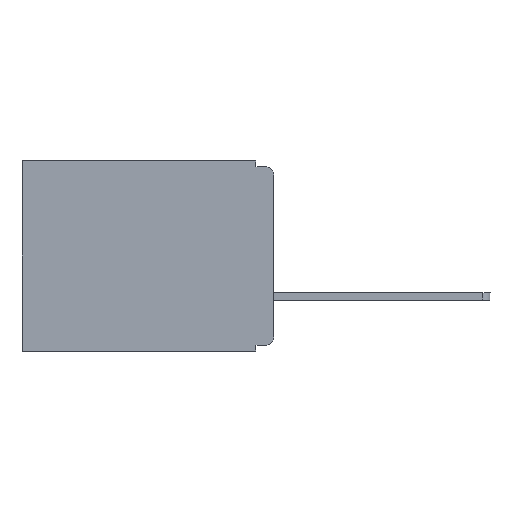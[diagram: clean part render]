
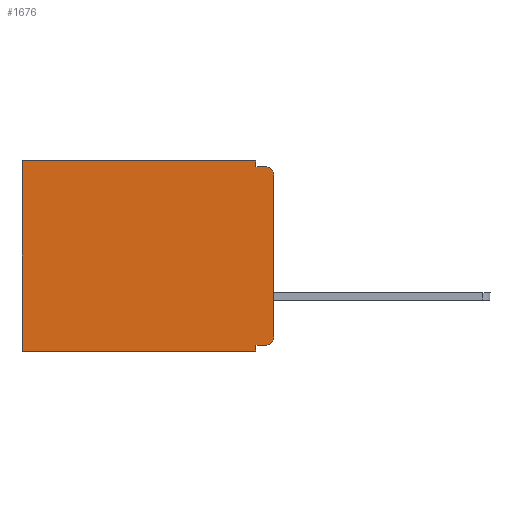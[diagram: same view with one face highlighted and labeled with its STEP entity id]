
A CAD part, left-side view. The second image highlights one B-rep face of the part: STEP entity #1676.
In plain terms, the highlighted planar face has unit normal (-1, 0, 0).
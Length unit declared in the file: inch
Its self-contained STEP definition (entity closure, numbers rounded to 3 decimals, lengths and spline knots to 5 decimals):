
#54 = CARTESIAN_POINT ( 'NONE',  ( 0.3, 0., -0.33 ) ) ;
#167 = VERTEX_POINT ( 'NONE', #6748 ) ;
#333 = VECTOR ( 'NONE', #10837, 39.37008 ) ;
#341 = PLANE ( 'NONE',  #2718 ) ;
#878 = DIRECTION ( 'NONE',  ( 0., 1., 0. ) ) ;
#884 = VECTOR ( 'NONE', #2899, 39.37008 ) ;
#930 = EDGE_CURVE ( 'NONE', #6573, #12989, #11190, .T. ) ;
#1018 = ORIENTED_EDGE ( 'NONE', *, *, #9528, .T. ) ;
#1331 = VERTEX_POINT ( 'NONE', #4767 ) ;
#1585 = EDGE_CURVE ( 'NONE', #167, #3086, #12884, .T. ) ;
#1676 = ADVANCED_FACE ( 'NONE', ( #2302 ), #341, .F. ) ;
#2039 = ORIENTED_EDGE ( 'NONE', *, *, #930, .T. ) ;
#2302 = FACE_OUTER_BOUND ( 'NONE', #2448, .T. ) ;
#2439 = CIRCLE ( 'NONE', #5686, 0.015 ) ;
#2448 = EDGE_LOOP ( 'NONE', ( #11182, #5757, #12698, #13178, #2039, #1018, #11456, #3758, #7376, #3087 ) ) ;
#2454 = LINE ( 'NONE', #13565, #10683 ) ;
#2503 = EDGE_CURVE ( 'NONE', #13521, #1331, #2439, .T. ) ;
#2718 = AXIS2_PLACEMENT_3D ( 'NONE', #3379, #8680, #5554 ) ;
#2777 = DIRECTION ( 'NONE',  ( 0., 1., 0. ) ) ;
#2899 = DIRECTION ( 'NONE',  ( 0., -1., 0. ) ) ;
#3066 = AXIS2_PLACEMENT_3D ( 'NONE', #4634, #8863, #5655 ) ;
#3086 = VERTEX_POINT ( 'NONE', #11547 ) ;
#3087 = ORIENTED_EDGE ( 'NONE', *, *, #10716, .T. ) ;
#3252 = VERTEX_POINT ( 'NONE', #3298 ) ;
#3274 = CARTESIAN_POINT ( 'NONE',  ( 0.3, 0., -0.32 ) ) ;
#3298 = CARTESIAN_POINT ( 'NONE',  ( 0.3, 0., -0.305 ) ) ;
#3379 = CARTESIAN_POINT ( 'NONE',  ( 0.3, 0., -0.33 ) ) ;
#3758 = ORIENTED_EDGE ( 'NONE', *, *, #9225, .F. ) ;
#3961 = DIRECTION ( 'NONE',  ( 0., 0., -1. ) ) ;
#4039 = VECTOR ( 'NONE', #7581, 39.37008 ) ;
#4058 = EDGE_CURVE ( 'NONE', #9631, #13279, #10484, .T. ) ;
#4242 = CARTESIAN_POINT ( 'NONE',  ( 0.3, 0.015, -0.32 ) ) ;
#4634 = CARTESIAN_POINT ( 'NONE',  ( 0.3, 0.015, -0.305 ) ) ;
#4767 = CARTESIAN_POINT ( 'NONE',  ( 0.3, 0.015, -0.01 ) ) ;
#5142 = DIRECTION ( 'NONE',  ( 0., 0., -1. ) ) ;
#5554 = DIRECTION ( 'NONE',  ( 0., 0., -1. ) ) ;
#5655 = DIRECTION ( 'NONE',  ( 0., 0., -1. ) ) ;
#5686 = AXIS2_PLACEMENT_3D ( 'NONE', #9345, #12616, #5142 ) ;
#5718 = LINE ( 'NONE', #9751, #333 ) ;
#5719 = EDGE_CURVE ( 'NONE', #13521, #3252, #5801, .T. ) ;
#5757 = ORIENTED_EDGE ( 'NONE', *, *, #2503, .T. ) ;
#5801 = LINE ( 'NONE', #12309, #12481 ) ;
#6573 = VERTEX_POINT ( 'NONE', #9474 ) ;
#6748 = CARTESIAN_POINT ( 'NONE',  ( 0.3, 0.031, -0.33 ) ) ;
#7028 = CARTESIAN_POINT ( 'NONE',  ( 0.3, 0., 0. ) ) ;
#7119 = CARTESIAN_POINT ( 'NONE',  ( 0.3, 0.031, -0.33 ) ) ;
#7376 = ORIENTED_EDGE ( 'NONE', *, *, #4058, .F. ) ;
#7581 = DIRECTION ( 'NONE',  ( 0., 1., 0. ) ) ;
#7694 = VECTOR ( 'NONE', #10403, 39.37008 ) ;
#8056 = EDGE_CURVE ( 'NONE', #11805, #1331, #10870, .T. ) ;
#8240 = VECTOR ( 'NONE', #2777, 39.37008 ) ;
#8373 = CIRCLE ( 'NONE', #3066, 0.015 ) ;
#8680 = DIRECTION ( 'NONE',  ( 1., 0., 0. ) ) ;
#8752 = CARTESIAN_POINT ( 'NONE',  ( 0.3, 0.437, 0. ) ) ;
#8863 = DIRECTION ( 'NONE',  ( -1., 0., 0. ) ) ;
#9077 = DIRECTION ( 'NONE',  ( 0., 0., -1. ) ) ;
#9225 = EDGE_CURVE ( 'NONE', #13279, #167, #12386, .T. ) ;
#9345 = CARTESIAN_POINT ( 'NONE',  ( 0.3, 0.015, -0.025 ) ) ;
#9474 = CARTESIAN_POINT ( 'NONE',  ( 0.3, 0.031, 0. ) ) ;
#9528 = EDGE_CURVE ( 'NONE', #12989, #3086, #2454, .T. ) ;
#9631 = VERTEX_POINT ( 'NONE', #4242 ) ;
#9751 = CARTESIAN_POINT ( 'NONE',  ( 0.3, 0.031, 0. ) ) ;
#10403 = DIRECTION ( 'NONE',  ( 0., 0., -1. ) ) ;
#10484 = LINE ( 'NONE', #3274, #4039 ) ;
#10683 = VECTOR ( 'NONE', #3961, 39.37008 ) ;
#10691 = EDGE_CURVE ( 'NONE', #6573, #11805, #5718, .T. ) ;
#10716 = EDGE_CURVE ( 'NONE', #9631, #3252, #8373, .T. ) ;
#10837 = DIRECTION ( 'NONE',  ( 0., 0., -1. ) ) ;
#10870 = LINE ( 'NONE', #13680, #884 ) ;
#11182 = ORIENTED_EDGE ( 'NONE', *, *, #5719, .F. ) ;
#11190 = LINE ( 'NONE', #7028, #8240 ) ;
#11456 = ORIENTED_EDGE ( 'NONE', *, *, #1585, .F. ) ;
#11547 = CARTESIAN_POINT ( 'NONE',  ( 0.3, 0.437, -0.33 ) ) ;
#11805 = VERTEX_POINT ( 'NONE', #13422 ) ;
#12309 = CARTESIAN_POINT ( 'NONE',  ( 0.3, 0., -0.33 ) ) ;
#12386 = LINE ( 'NONE', #7119, #7694 ) ;
#12481 = VECTOR ( 'NONE', #9077, 39.37008 ) ;
#12554 = VECTOR ( 'NONE', #878, 39.37008 ) ;
#12616 = DIRECTION ( 'NONE',  ( -1., 0., 0. ) ) ;
#12698 = ORIENTED_EDGE ( 'NONE', *, *, #8056, .F. ) ;
#12729 = CARTESIAN_POINT ( 'NONE',  ( 0.3, 0., -0.025 ) ) ;
#12742 = CARTESIAN_POINT ( 'NONE',  ( 0.3, 0.031, -0.32 ) ) ;
#12884 = LINE ( 'NONE', #54, #12554 ) ;
#12989 = VERTEX_POINT ( 'NONE', #8752 ) ;
#13178 = ORIENTED_EDGE ( 'NONE', *, *, #10691, .F. ) ;
#13279 = VERTEX_POINT ( 'NONE', #12742 ) ;
#13422 = CARTESIAN_POINT ( 'NONE',  ( 0.3, 0.031, -0.01 ) ) ;
#13521 = VERTEX_POINT ( 'NONE', #12729 ) ;
#13565 = CARTESIAN_POINT ( 'NONE',  ( 0.3, 0.437, -0.33 ) ) ;
#13680 = CARTESIAN_POINT ( 'NONE',  ( 0.3, 0., -0.01 ) ) ;
